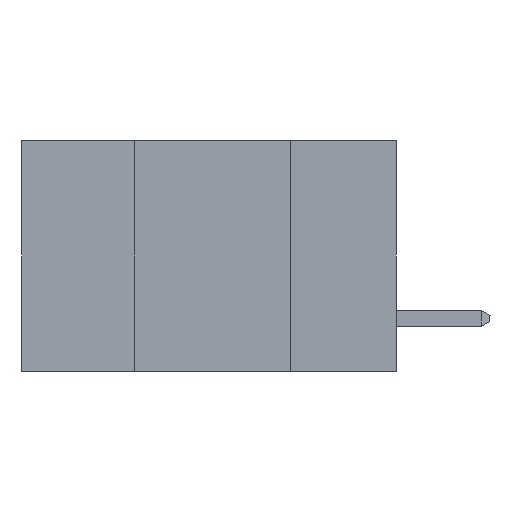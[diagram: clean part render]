
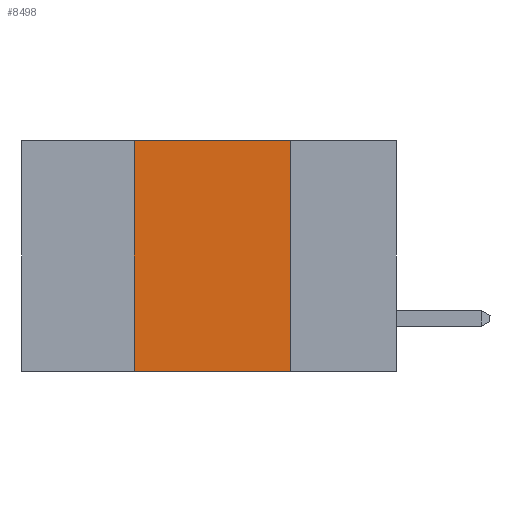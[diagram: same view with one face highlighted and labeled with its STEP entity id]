
A CAD part, left-side view. The second image highlights one B-rep face of the part: STEP entity #8498.
In plain terms, the highlighted planar face has unit normal (-1, 0, 0).
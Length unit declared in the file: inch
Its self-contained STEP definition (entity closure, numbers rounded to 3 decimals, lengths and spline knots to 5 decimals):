
#694 = LINE ( 'NONE', #1170, #15138 ) ;
#840 = CARTESIAN_POINT ( 'NONE',  ( 0., 0.6, 0. ) ) ;
#856 = ORIENTED_EDGE ( 'NONE', *, *, #8490, .F. ) ;
#909 = CARTESIAN_POINT ( 'NONE',  ( 0., 0.42, 0. ) ) ;
#963 = PLANE ( 'NONE',  #5658 ) ;
#1170 = CARTESIAN_POINT ( 'NONE',  ( 0., 0.17, -0.37 ) ) ;
#1610 = VERTEX_POINT ( 'NONE', #5483 ) ;
#1900 = DIRECTION ( 'NONE',  ( 0., 0., 1. ) ) ;
#2096 = EDGE_CURVE ( 'NONE', #13796, #4301, #13444, .T. ) ;
#3809 = CARTESIAN_POINT ( 'NONE',  ( 0., 0.17, -0.37 ) ) ;
#4114 = CARTESIAN_POINT ( 'NONE',  ( 0., 0.6, -0.37 ) ) ;
#4301 = VERTEX_POINT ( 'NONE', #909 ) ;
#5455 = CARTESIAN_POINT ( 'NONE',  ( 0., 0.42, -0.37 ) ) ;
#5483 = CARTESIAN_POINT ( 'NONE',  ( 0., 0.17, 0. ) ) ;
#5658 = AXIS2_PLACEMENT_3D ( 'NONE', #840, #23181, #22918 ) ;
#5990 = EDGE_CURVE ( 'NONE', #4301, #1610, #6777, .T. ) ;
#6502 = ORIENTED_EDGE ( 'NONE', *, *, #5990, .F. ) ;
#6777 = LINE ( 'NONE', #13915, #16136 ) ;
#8332 = LINE ( 'NONE', #4114, #13354 ) ;
#8435 = VECTOR ( 'NONE', #1900, 39.37008 ) ;
#8490 = EDGE_CURVE ( 'NONE', #1610, #16882, #694, .T. ) ;
#8498 = ADVANCED_FACE ( 'NONE', ( #19987 ), #963, .F. ) ;
#10325 = DIRECTION ( 'NONE',  ( 0., 0., -1. ) ) ;
#10571 = CARTESIAN_POINT ( 'NONE',  ( 0., 0.42, -0.37 ) ) ;
#11516 = ORIENTED_EDGE ( 'NONE', *, *, #2096, .F. ) ;
#12121 = EDGE_LOOP ( 'NONE', ( #856, #6502, #11516, #16443 ) ) ;
#13354 = VECTOR ( 'NONE', #13559, 39.37008 ) ;
#13444 = LINE ( 'NONE', #5455, #8435 ) ;
#13559 = DIRECTION ( 'NONE',  ( 0., -1., 0. ) ) ;
#13796 = VERTEX_POINT ( 'NONE', #10571 ) ;
#13864 = DIRECTION ( 'NONE',  ( 0., -1., 0. ) ) ;
#13915 = CARTESIAN_POINT ( 'NONE',  ( 0., 0.6, 0. ) ) ;
#15138 = VECTOR ( 'NONE', #10325, 39.37008 ) ;
#16136 = VECTOR ( 'NONE', #13864, 39.37008 ) ;
#16443 = ORIENTED_EDGE ( 'NONE', *, *, #23615, .T. ) ;
#16882 = VERTEX_POINT ( 'NONE', #3809 ) ;
#19987 = FACE_OUTER_BOUND ( 'NONE', #12121, .T. ) ;
#22918 = DIRECTION ( 'NONE',  ( 0., 0., -1. ) ) ;
#23181 = DIRECTION ( 'NONE',  ( 1., 0., 0. ) ) ;
#23615 = EDGE_CURVE ( 'NONE', #13796, #16882, #8332, .T. ) ;
